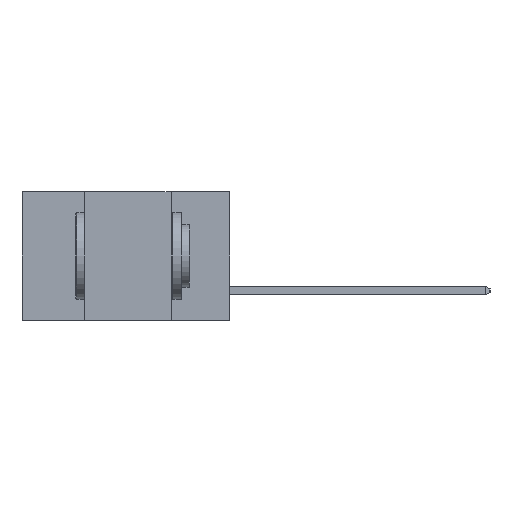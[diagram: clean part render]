
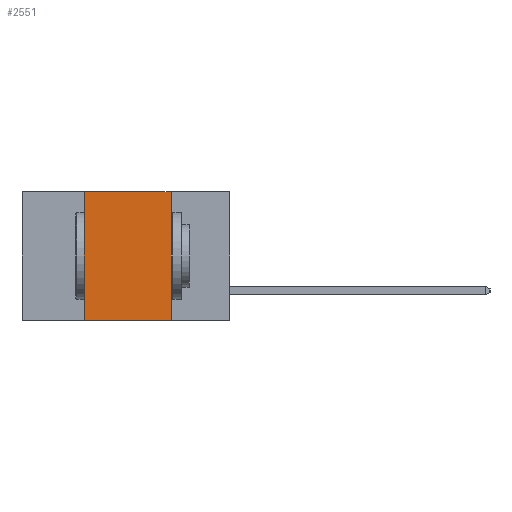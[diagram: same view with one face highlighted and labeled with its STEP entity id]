
A CAD part, left-side view. The second image highlights one B-rep face of the part: STEP entity #2551.
In plain terms, the highlighted planar face has unit normal (-1, 0, 0).
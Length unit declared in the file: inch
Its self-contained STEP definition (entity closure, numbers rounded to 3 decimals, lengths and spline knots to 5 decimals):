
#1812 = CARTESIAN_POINT ( 'NONE',  ( 0., 0.42, 0. ) ) ;
#1922 = VECTOR ( 'NONE', #8012, 39.37008 ) ;
#2114 = EDGE_LOOP ( 'NONE', ( #4343, #17735, #7808, #11526 ) ) ;
#2336 = AXIS2_PLACEMENT_3D ( 'NONE', #5149, #19389, #20074 ) ;
#2409 = LINE ( 'NONE', #4625, #10479 ) ;
#2551 = ADVANCED_FACE ( 'NONE', ( #4125 ), #20143, .F. ) ;
#3777 = DIRECTION ( 'NONE',  ( 0., 0., 1. ) ) ;
#4125 = FACE_OUTER_BOUND ( 'NONE', #2114, .T. ) ;
#4198 = CARTESIAN_POINT ( 'NONE',  ( 0., 0.17, -0.37 ) ) ;
#4343 = ORIENTED_EDGE ( 'NONE', *, *, #20625, .F. ) ;
#4447 = VERTEX_POINT ( 'NONE', #4198 ) ;
#4625 = CARTESIAN_POINT ( 'NONE',  ( 0., 0.17, 0. ) ) ;
#5149 = CARTESIAN_POINT ( 'NONE',  ( 0., 0.6, 0. ) ) ;
#6263 = DIRECTION ( 'NONE',  ( 0., 0., -1. ) ) ;
#7808 = ORIENTED_EDGE ( 'NONE', *, *, #20872, .F. ) ;
#8012 = DIRECTION ( 'NONE',  ( 0., -1., 0. ) ) ;
#8049 = DIRECTION ( 'NONE',  ( 0., -1., 0. ) ) ;
#9327 = VERTEX_POINT ( 'NONE', #1812 ) ;
#9729 = VECTOR ( 'NONE', #3777, 39.37008 ) ;
#9997 = CARTESIAN_POINT ( 'NONE',  ( 0., 0.17, 0. ) ) ;
#10233 = LINE ( 'NONE', #11850, #9729 ) ;
#10479 = VECTOR ( 'NONE', #6263, 39.37008 ) ;
#11294 = CARTESIAN_POINT ( 'NONE',  ( 0., 0.6, 0. ) ) ;
#11526 = ORIENTED_EDGE ( 'NONE', *, *, #18810, .T. ) ;
#11648 = VERTEX_POINT ( 'NONE', #12870 ) ;
#11850 = CARTESIAN_POINT ( 'NONE',  ( 0., 0.42, 0. ) ) ;
#12870 = CARTESIAN_POINT ( 'NONE',  ( 0., 0.42, -0.37 ) ) ;
#16146 = CARTESIAN_POINT ( 'NONE',  ( 0., 0.6, -0.37 ) ) ;
#16983 = VECTOR ( 'NONE', #8049, 39.37008 ) ;
#17479 = EDGE_CURVE ( 'NONE', #9327, #18319, #17505, .T. ) ;
#17505 = LINE ( 'NONE', #11294, #16983 ) ;
#17735 = ORIENTED_EDGE ( 'NONE', *, *, #17479, .F. ) ;
#18319 = VERTEX_POINT ( 'NONE', #9997 ) ;
#18810 = EDGE_CURVE ( 'NONE', #11648, #4447, #19167, .T. ) ;
#19167 = LINE ( 'NONE', #16146, #1922 ) ;
#19389 = DIRECTION ( 'NONE',  ( 1., 0., 0. ) ) ;
#20074 = DIRECTION ( 'NONE',  ( 0., 0., -1. ) ) ;
#20143 = PLANE ( 'NONE',  #2336 ) ;
#20625 = EDGE_CURVE ( 'NONE', #18319, #4447, #2409, .T. ) ;
#20872 = EDGE_CURVE ( 'NONE', #11648, #9327, #10233, .T. ) ;
